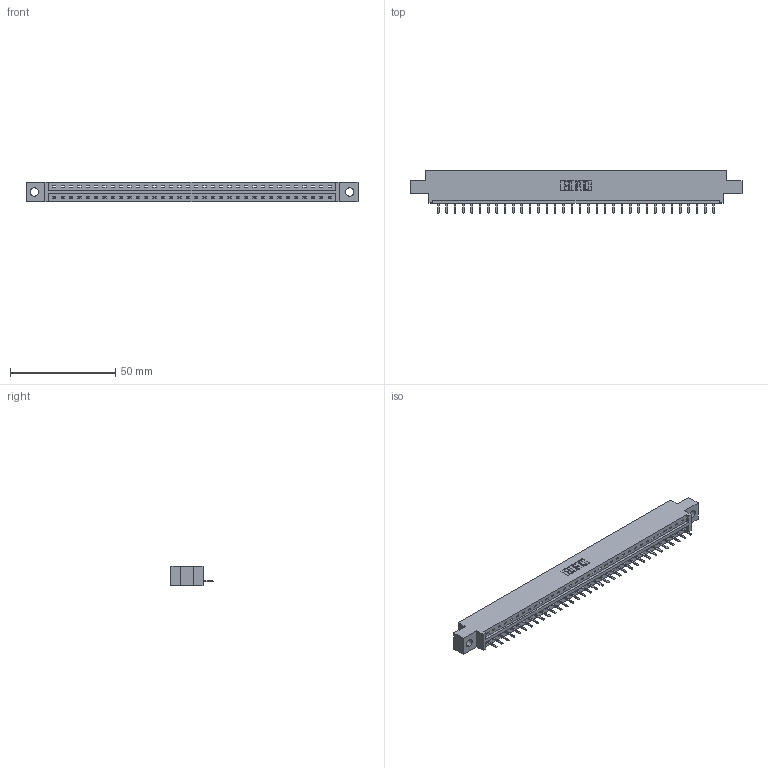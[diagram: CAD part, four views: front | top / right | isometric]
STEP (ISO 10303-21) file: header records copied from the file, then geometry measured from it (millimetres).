
FILE_DESCRIPTION (( 'STEP AP203' ), '1' );
FILE_NAME ('337-034-520-604.STEP', '2019-10-01T11:24:56', ( '' ), ( '' ), 'SwSTEP 2.0', 'SolidWorks 2016', '' );
FILE_SCHEMA (( 'CONFIG_CONTROL_DESIGN' ));
Length unit declared in the file: inch
Products named in the file (3): 337 Part_0.170 Offset - 0.156 Dia-TH; 337-034-520-604; 345-292-001_345-293-120
Assembly tree (35 placements, depth 2):
  337-034-520-604
    337 Part_0.170 Offset - 0.156 Dia-TH
    345-292-001_345-293-120  x34
Bounding box: 157.73 x 20.02 x 9.4 mm (x, y, z)
Volume: 15990.5 mm3; surface area: 16019.1 mm2
Topology: 35 solids, 35 shells, 2362 faces, 6987 edges, 4566 vertices
Faces by surface type: plane 1706, cylinder 656
Entity records: 26557 total; most frequent: CARTESIAN_POINT 4644, ORIENTED_EDGE 4602, DIRECTION 3913, EDGE_CURVE 2301, VECTOR 2169, LINE 2169, VERTEX_POINT 1530, AXIS2_PLACEMENT_3D 872
